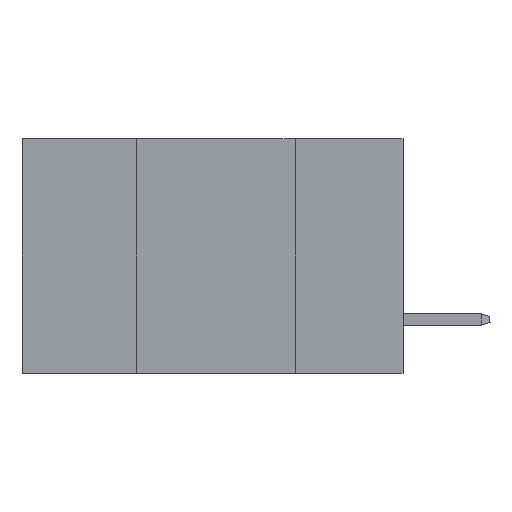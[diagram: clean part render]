
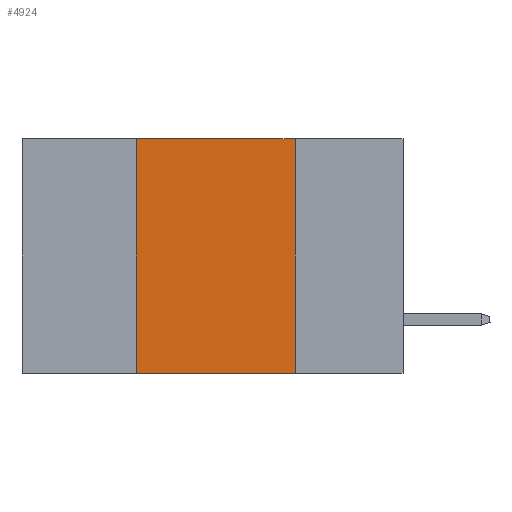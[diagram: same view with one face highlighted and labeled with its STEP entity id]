
A CAD part, left-side view. The second image highlights one B-rep face of the part: STEP entity #4924.
In plain terms, the highlighted planar face has unit normal (-1, 0, 0).
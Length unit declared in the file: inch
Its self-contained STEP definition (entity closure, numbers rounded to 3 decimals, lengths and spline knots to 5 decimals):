
#306 = DIRECTION ( 'NONE',  ( 0., -1., 0. ) ) ;
#1432 = AXIS2_PLACEMENT_3D ( 'NONE', #21861, #16191, #4575 ) ;
#3063 = PLANE ( 'NONE',  #1432 ) ;
#3070 = ORIENTED_EDGE ( 'NONE', *, *, #23610, .T. ) ;
#4508 = LINE ( 'NONE', #13859, #15603 ) ;
#4518 = VERTEX_POINT ( 'NONE', #17774 ) ;
#4575 = DIRECTION ( 'NONE',  ( 0., 0., -1. ) ) ;
#4924 = ADVANCED_FACE ( 'NONE', ( #18087 ), #3063, .F. ) ;
#6911 = EDGE_CURVE ( 'NONE', #15619, #8582, #4508, .T. ) ;
#7094 = CARTESIAN_POINT ( 'NONE',  ( 0., 0.42, -0.37 ) ) ;
#7775 = EDGE_CURVE ( 'NONE', #8582, #4518, #14167, .T. ) ;
#8582 = VERTEX_POINT ( 'NONE', #21765 ) ;
#8621 = VECTOR ( 'NONE', #15177, 39.37008 ) ;
#12273 = CARTESIAN_POINT ( 'NONE',  ( 0., 0.6, 0. ) ) ;
#13035 = LINE ( 'NONE', #22877, #8621 ) ;
#13859 = CARTESIAN_POINT ( 'NONE',  ( 0., 0.42, 0. ) ) ;
#14167 = LINE ( 'NONE', #12273, #14438 ) ;
#14438 = VECTOR ( 'NONE', #21854, 39.37008 ) ;
#15177 = DIRECTION ( 'NONE',  ( 0., 0., -1. ) ) ;
#15603 = VECTOR ( 'NONE', #16132, 39.37008 ) ;
#15619 = VERTEX_POINT ( 'NONE', #7094 ) ;
#16132 = DIRECTION ( 'NONE',  ( 0., 0., 1. ) ) ;
#16191 = DIRECTION ( 'NONE',  ( 1., 0., 0. ) ) ;
#17024 = EDGE_CURVE ( 'NONE', #4518, #19319, #13035, .T. ) ;
#17608 = CARTESIAN_POINT ( 'NONE',  ( 0., 0.6, -0.37 ) ) ;
#17774 = CARTESIAN_POINT ( 'NONE',  ( 0., 0.17, 0. ) ) ;
#18087 = FACE_OUTER_BOUND ( 'NONE', #24716, .T. ) ;
#18506 = ORIENTED_EDGE ( 'NONE', *, *, #6911, .F. ) ;
#18943 = ORIENTED_EDGE ( 'NONE', *, *, #17024, .F. ) ;
#19319 = VERTEX_POINT ( 'NONE', #22446 ) ;
#19661 = VECTOR ( 'NONE', #306, 39.37008 ) ;
#21636 = LINE ( 'NONE', #17608, #19661 ) ;
#21765 = CARTESIAN_POINT ( 'NONE',  ( 0., 0.42, 0. ) ) ;
#21854 = DIRECTION ( 'NONE',  ( 0., -1., 0. ) ) ;
#21861 = CARTESIAN_POINT ( 'NONE',  ( 0., 0.6, 0. ) ) ;
#22446 = CARTESIAN_POINT ( 'NONE',  ( 0., 0.17, -0.37 ) ) ;
#22877 = CARTESIAN_POINT ( 'NONE',  ( 0., 0.17, 0. ) ) ;
#23610 = EDGE_CURVE ( 'NONE', #15619, #19319, #21636, .T. ) ;
#24716 = EDGE_LOOP ( 'NONE', ( #18943, #24806, #18506, #3070 ) ) ;
#24806 = ORIENTED_EDGE ( 'NONE', *, *, #7775, .F. ) ;
